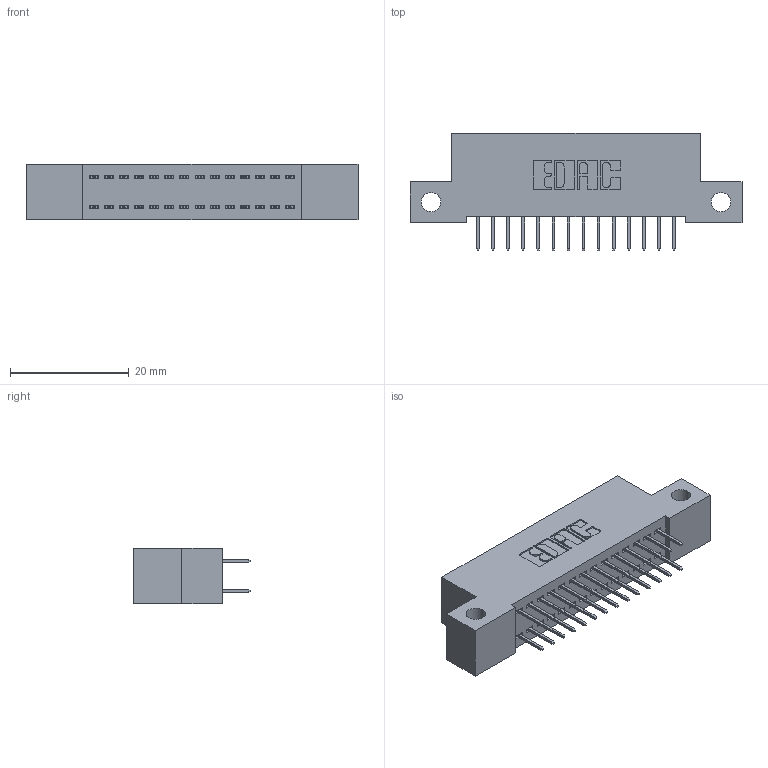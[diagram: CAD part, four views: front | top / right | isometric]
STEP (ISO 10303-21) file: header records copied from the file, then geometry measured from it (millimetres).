
FILE_DESCRIPTION (( 'STEP AP203' ), '1' );
FILE_NAME ('392-028-524-212.STEP', '2018-08-15T21:00:34', ( '' ), ( '' ), 'SwSTEP 2.0', 'SolidWorks 2016', '' );
FILE_SCHEMA (( 'CONFIG_CONTROL_DESIGN' ));
Length unit declared in the file: inch
Products named in the file (3): 342 Part_Side Mount; 345-292-001_345-293-124; 392-028-524-212
Assembly tree (29 placements, depth 2):
  392-028-524-212
    342 Part_Side Mount
    345-292-001_345-293-124  x28
Bounding box: 55.88 x 19.69 x 9.4 mm (x, y, z)
Volume: 4772 mm3; surface area: 6807.7 mm2
Topology: 29 solids, 29 shells, 1678 faces, 4751 edges, 3054 vertices
Faces by surface type: plane 1242, cylinder 436
Entity records: 12573 total; most frequent: CARTESIAN_POINT 2114, ORIENTED_EDGE 2050, DIRECTION 1857, EDGE_CURVE 1025, LINE 901, VECTOR 901, VERTEX_POINT 678, AXIS2_PLACEMENT_3D 478
